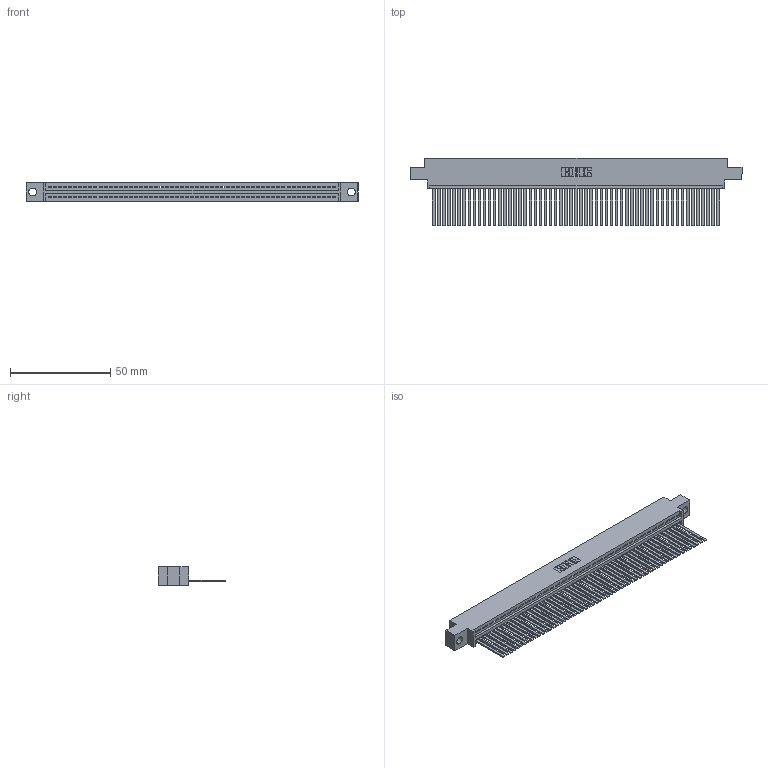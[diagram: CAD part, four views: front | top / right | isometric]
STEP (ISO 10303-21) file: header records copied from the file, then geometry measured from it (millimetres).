
FILE_DESCRIPTION (( 'STEP AP203' ), '1' );
FILE_NAME ('345-057-544-604.STEP', '2018-09-21T11:32:08', ( '' ), ( '' ), 'SwSTEP 2.0', 'SolidWorks 2016', '' );
FILE_SCHEMA (( 'CONFIG_CONTROL_DESIGN' ));
Length unit declared in the file: inch
Products named in the file (3): 345 Part_0.170 Offset - 0.156 Dia-TH; 345-292-001_345-293-144; 345-057-544-604
Assembly tree (58 placements, depth 2):
  345-057-544-604
    345 Part_0.170 Offset - 0.156 Dia-TH
    345-292-001_345-293-144  x57
Bounding box: 165.99 x 33.96 x 9.4 mm (x, y, z)
Volume: 16347.6 mm3; surface area: 23845.4 mm2
Topology: 58 solids, 58 shells, 3094 faces, 9359 edges, 6162 vertices
Faces by surface type: plane 2136, cylinder 958
Entity records: 40831 total; most frequent: CARTESIAN_POINT 7079, ORIENTED_EDGE 7070, DIRECTION 6157, EDGE_CURVE 3535, LINE 3179, VECTOR 3179, VERTEX_POINT 2354, AXIS2_PLACEMENT_3D 1489
